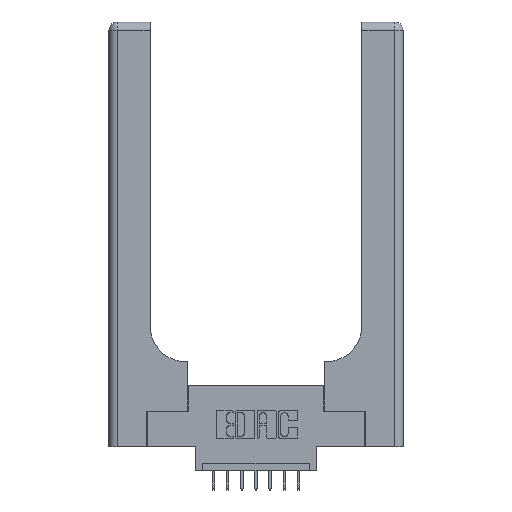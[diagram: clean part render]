
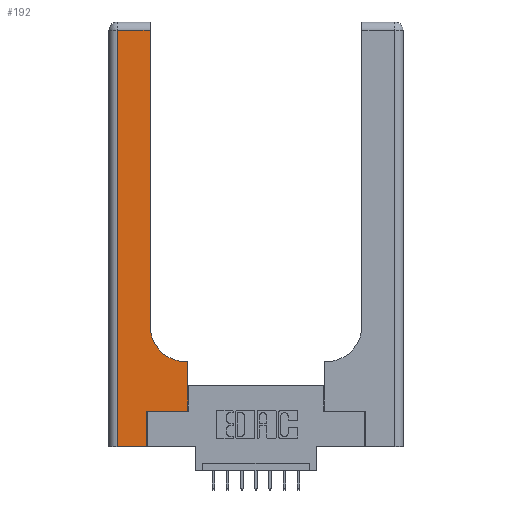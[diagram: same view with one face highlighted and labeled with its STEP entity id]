
A CAD part, top view. The second image highlights one B-rep face of the part: STEP entity #192.
In plain terms, the highlighted planar face has unit normal (0, 0, 1).
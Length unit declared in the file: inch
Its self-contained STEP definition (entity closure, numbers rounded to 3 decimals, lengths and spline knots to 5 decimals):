
#55 = ORIENTED_EDGE ( 'NONE', *, *, #9142, .T. ) ;
#179 = CARTESIAN_POINT ( 'NONE',  ( 0.06, 2.94, 0.37 ) ) ;
#192 = ADVANCED_FACE ( 'NONE', ( #3808 ), #2638, .F. ) ;
#477 = CARTESIAN_POINT ( 'NONE',  ( 0.2915, 0.85, 0.37 ) ) ;
#842 = CARTESIAN_POINT ( 'NONE',  ( 0.06, 3., 0.37 ) ) ;
#905 = VECTOR ( 'NONE', #2304, 39.37008 ) ;
#996 = CARTESIAN_POINT ( 'NONE',  ( 0.2915, 0.6, 0.37 ) ) ;
#1112 = CARTESIAN_POINT ( 'NONE',  ( 0.2915, 3., 0.37 ) ) ;
#1194 = VECTOR ( 'NONE', #10289, 39.37008 ) ;
#1215 = EDGE_CURVE ( 'NONE', #2138, #14055, #15017, .T. ) ;
#1465 = DIRECTION ( 'NONE',  ( 0., 0., -1. ) ) ;
#1944 = DIRECTION ( 'NONE',  ( 0., -1., 0. ) ) ;
#2048 = CARTESIAN_POINT ( 'NONE',  ( 0., 2.94, 0.37 ) ) ;
#2138 = VERTEX_POINT ( 'NONE', #11145 ) ;
#2278 = DIRECTION ( 'NONE',  ( 0., 1., 0. ) ) ;
#2304 = DIRECTION ( 'NONE',  ( -1., 0., 0. ) ) ;
#2351 = LINE ( 'NONE', #2048, #6138 ) ;
#2638 = PLANE ( 'NONE',  #3436 ) ;
#3005 = CARTESIAN_POINT ( 'NONE',  ( 0.5585, 0.25, 0.37 ) ) ;
#3270 = LINE ( 'NONE', #7938, #1194 ) ;
#3436 = AXIS2_PLACEMENT_3D ( 'NONE', #3888, #1465, #8613 ) ;
#3695 = VERTEX_POINT ( 'NONE', #477 ) ;
#3808 = FACE_OUTER_BOUND ( 'NONE', #7818, .T. ) ;
#3888 = CARTESIAN_POINT ( 'NONE',  ( 0., 3., 0.37 ) ) ;
#4059 = ORIENTED_EDGE ( 'NONE', *, *, #8662, .T. ) ;
#4200 = ORIENTED_EDGE ( 'NONE', *, *, #14151, .T. ) ;
#4324 = VECTOR ( 'NONE', #13275, 39.37008 ) ;
#4456 = DIRECTION ( 'NONE',  ( 0., 1., 0. ) ) ;
#4567 = CARTESIAN_POINT ( 'NONE',  ( 0.5415, 0.85, 0.37 ) ) ;
#5110 = VERTEX_POINT ( 'NONE', #11364 ) ;
#5593 = EDGE_CURVE ( 'NONE', #15353, #14362, #9477, .T. ) ;
#5718 = ORIENTED_EDGE ( 'NONE', *, *, #15111, .T. ) ;
#5890 = CARTESIAN_POINT ( 'NONE',  ( 0.5585, 0.6, 0.37 ) ) ;
#6068 = CIRCLE ( 'NONE', #11782, 0.25 ) ;
#6138 = VECTOR ( 'NONE', #15349, 39.37008 ) ;
#6259 = ORIENTED_EDGE ( 'NONE', *, *, #9462, .T. ) ;
#7352 = ORIENTED_EDGE ( 'NONE', *, *, #11400, .T. ) ;
#7604 = ORIENTED_EDGE ( 'NONE', *, *, #5593, .T. ) ;
#7672 = VERTEX_POINT ( 'NONE', #179 ) ;
#7818 = EDGE_LOOP ( 'NONE', ( #5718, #4059, #6259, #4200, #12026, #13341, #55, #7604, #7352 ) ) ;
#7938 = CARTESIAN_POINT ( 'NONE',  ( 0.269, 0.25, 0.37 ) ) ;
#8086 = DIRECTION ( 'NONE',  ( 0., 1., 0. ) ) ;
#8275 = VECTOR ( 'NONE', #2278, 39.37008 ) ;
#8613 = DIRECTION ( 'NONE',  ( -1., 0., 0. ) ) ;
#8662 = EDGE_CURVE ( 'NONE', #5110, #7672, #2351, .T. ) ;
#9142 = EDGE_CURVE ( 'NONE', #9808, #15353, #13989, .T. ) ;
#9315 = DIRECTION ( 'NONE',  ( 1., 0., 0. ) ) ;
#9385 = VECTOR ( 'NONE', #4456, 39.37008 ) ;
#9462 = EDGE_CURVE ( 'NONE', #7672, #13776, #12590, .T. ) ;
#9477 = LINE ( 'NONE', #996, #905 ) ;
#9730 = VECTOR ( 'NONE', #8086, 39.37008 ) ;
#9808 = VERTEX_POINT ( 'NONE', #3005 ) ;
#10029 = CARTESIAN_POINT ( 'NONE',  ( 0.5415, 0.6, 0.37 ) ) ;
#10289 = DIRECTION ( 'NONE',  ( 1., 0., 0. ) ) ;
#10434 = CARTESIAN_POINT ( 'NONE',  ( 0.06, 0., 0.37 ) ) ;
#10887 = LINE ( 'NONE', #13047, #4324 ) ;
#11145 = CARTESIAN_POINT ( 'NONE',  ( 0.269, 0., 0.37 ) ) ;
#11364 = CARTESIAN_POINT ( 'NONE',  ( 0.2915, 2.94, 0.37 ) ) ;
#11375 = VECTOR ( 'NONE', #1944, 39.37008 ) ;
#11400 = EDGE_CURVE ( 'NONE', #14362, #3695, #6068, .T. ) ;
#11782 = AXIS2_PLACEMENT_3D ( 'NONE', #4567, #13039, #9315 ) ;
#11986 = EDGE_CURVE ( 'NONE', #14055, #9808, #3270, .T. ) ;
#12026 = ORIENTED_EDGE ( 'NONE', *, *, #1215, .T. ) ;
#12590 = LINE ( 'NONE', #842, #11375 ) ;
#13004 = LINE ( 'NONE', #1112, #8275 ) ;
#13039 = DIRECTION ( 'NONE',  ( 0., 0., -1. ) ) ;
#13047 = CARTESIAN_POINT ( 'NONE',  ( 0., 0., 0.37 ) ) ;
#13275 = DIRECTION ( 'NONE',  ( 1., 0., 0. ) ) ;
#13341 = ORIENTED_EDGE ( 'NONE', *, *, #11986, .T. ) ;
#13776 = VERTEX_POINT ( 'NONE', #10434 ) ;
#13989 = LINE ( 'NONE', #15330, #9385 ) ;
#14055 = VERTEX_POINT ( 'NONE', #15310 ) ;
#14151 = EDGE_CURVE ( 'NONE', #13776, #2138, #10887, .T. ) ;
#14362 = VERTEX_POINT ( 'NONE', #10029 ) ;
#15017 = LINE ( 'NONE', #15169, #9730 ) ;
#15111 = EDGE_CURVE ( 'NONE', #3695, #5110, #13004, .T. ) ;
#15169 = CARTESIAN_POINT ( 'NONE',  ( 0.269, 0., 0.37 ) ) ;
#15310 = CARTESIAN_POINT ( 'NONE',  ( 0.269, 0.25, 0.37 ) ) ;
#15330 = CARTESIAN_POINT ( 'NONE',  ( 0.5585, 0.25, 0.37 ) ) ;
#15349 = DIRECTION ( 'NONE',  ( -1., 0., 0. ) ) ;
#15353 = VERTEX_POINT ( 'NONE', #5890 ) ;
